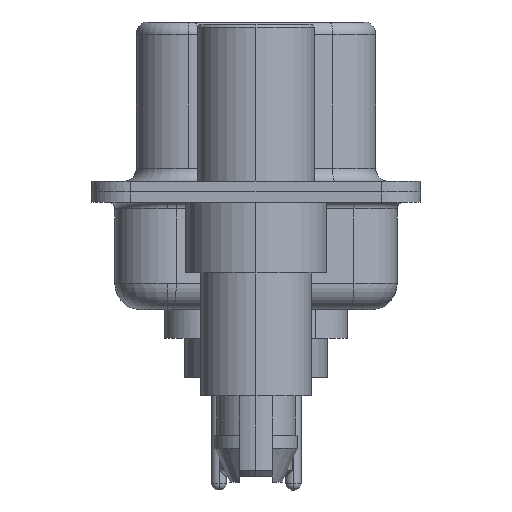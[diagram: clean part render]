
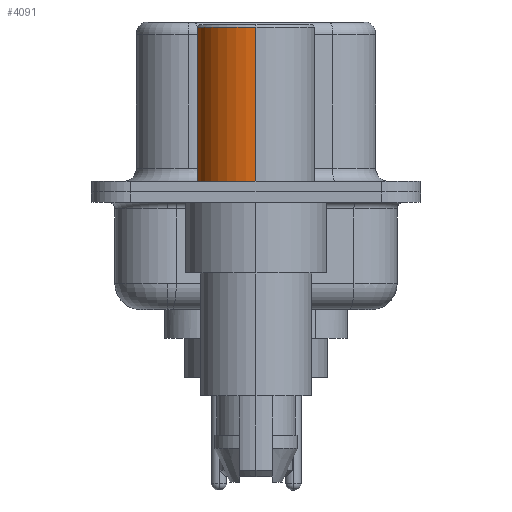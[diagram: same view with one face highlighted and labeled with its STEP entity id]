
A CAD part, left-side view. The second image highlights one B-rep face of the part: STEP entity #4091.
In plain terms, the highlighted cylindrical face has radius 2.25 mm (diameter 4.5 mm), a partial arc.
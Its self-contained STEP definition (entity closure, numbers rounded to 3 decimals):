
#699 = CARTESIAN_POINT ( 'NONE',  ( 2.25, 0., 0.4 ) ) ;
#857 = VERTEX_POINT ( 'NONE', #10258 ) ;
#1368 = ORIENTED_EDGE ( 'NONE', *, *, #11143, .F. ) ;
#1450 = EDGE_CURVE ( 'NONE', #5979, #9030, #9555, .T. ) ;
#1612 = CARTESIAN_POINT ( 'NONE',  ( 0., 0., 6.3 ) ) ;
#1675 = DIRECTION ( 'NONE',  ( 1., 0., 0. ) ) ;
#1751 = CIRCLE ( 'NONE', #9902, 2.25 ) ;
#2381 = CIRCLE ( 'NONE', #14767, 2.25 ) ;
#2624 = CARTESIAN_POINT ( 'NONE',  ( 0., 0., 0.581 ) ) ;
#3904 = DIRECTION ( 'NONE',  ( 1., 0., 0. ) ) ;
#4091 = ADVANCED_FACE ( 'NONE', ( #13319 ), #9922, .T. ) ;
#5440 = EDGE_LOOP ( 'NONE', ( #19194, #11241, #1368, #8797 ) ) ;
#5979 = VERTEX_POINT ( 'NONE', #699 ) ;
#7765 = EDGE_CURVE ( 'NONE', #5979, #14307, #1751, .T. ) ;
#8169 = CARTESIAN_POINT ( 'NONE',  ( 0., 0., 0.4 ) ) ;
#8797 = ORIENTED_EDGE ( 'NONE', *, *, #1450, .F. ) ;
#8876 = CARTESIAN_POINT ( 'NONE',  ( -2.25, 0., 0.4 ) ) ;
#9030 = VERTEX_POINT ( 'NONE', #18404 ) ;
#9555 = LINE ( 'NONE', #17791, #14155 ) ;
#9902 = AXIS2_PLACEMENT_3D ( 'NONE', #8169, #17272, #12664 ) ;
#9906 = VECTOR ( 'NONE', #12686, 1000. ) ;
#9922 = CYLINDRICAL_SURFACE ( 'NONE', #16703, 2.25 ) ;
#10062 = DIRECTION ( 'NONE',  ( 0., 0., 1. ) ) ;
#10258 = CARTESIAN_POINT ( 'NONE',  ( -2.25, 0., 6.3 ) ) ;
#10812 = DIRECTION ( 'NONE',  ( 0., 0., 1. ) ) ;
#11143 = EDGE_CURVE ( 'NONE', #9030, #857, #2381, .T. ) ;
#11241 = ORIENTED_EDGE ( 'NONE', *, *, #17021, .T. ) ;
#12439 = CARTESIAN_POINT ( 'NONE',  ( -2.25, 0., 0.581 ) ) ;
#12664 = DIRECTION ( 'NONE',  ( 1., 0., 0. ) ) ;
#12686 = DIRECTION ( 'NONE',  ( 0., 0., 1. ) ) ;
#13319 = FACE_OUTER_BOUND ( 'NONE', #5440, .T. ) ;
#14155 = VECTOR ( 'NONE', #16297, 1000. ) ;
#14307 = VERTEX_POINT ( 'NONE', #8876 ) ;
#14767 = AXIS2_PLACEMENT_3D ( 'NONE', #1612, #10812, #1675 ) ;
#16297 = DIRECTION ( 'NONE',  ( 0., 0., 1. ) ) ;
#16703 = AXIS2_PLACEMENT_3D ( 'NONE', #2624, #10062, #3904 ) ;
#17021 = EDGE_CURVE ( 'NONE', #14307, #857, #17156, .T. ) ;
#17156 = LINE ( 'NONE', #12439, #9906 ) ;
#17272 = DIRECTION ( 'NONE',  ( 0., 0., 1. ) ) ;
#17791 = CARTESIAN_POINT ( 'NONE',  ( 2.25, 0., 0.581 ) ) ;
#18404 = CARTESIAN_POINT ( 'NONE',  ( 2.25, 0., 6.3 ) ) ;
#19194 = ORIENTED_EDGE ( 'NONE', *, *, #7765, .T. ) ;
